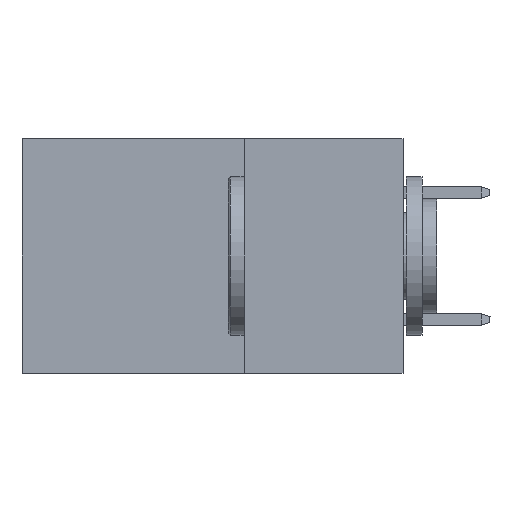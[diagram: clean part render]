
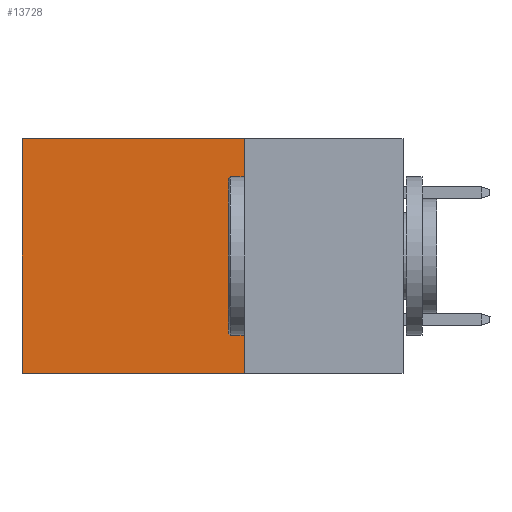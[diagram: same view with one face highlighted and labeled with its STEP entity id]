
A CAD part, left-side view. The second image highlights one B-rep face of the part: STEP entity #13728.
In plain terms, the highlighted planar face has unit normal (-1, 0, 0).
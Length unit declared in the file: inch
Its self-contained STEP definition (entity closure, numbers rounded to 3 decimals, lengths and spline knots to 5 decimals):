
#1766 = ORIENTED_EDGE ( 'NONE', *, *, #11098, .T. ) ;
#2034 = LINE ( 'NONE', #6676, #17856 ) ;
#2366 = ORIENTED_EDGE ( 'NONE', *, *, #22495, .F. ) ;
#5580 = VERTEX_POINT ( 'NONE', #10047 ) ;
#5663 = AXIS2_PLACEMENT_3D ( 'NONE', #6120, #18287, #27669 ) ;
#5741 = DIRECTION ( 'NONE',  ( 0., 1., 0. ) ) ;
#6120 = CARTESIAN_POINT ( 'NONE',  ( 0.2875, 0.25, 0. ) ) ;
#6676 = CARTESIAN_POINT ( 'NONE',  ( 0.2875, 0.6, 0. ) ) ;
#7139 = VECTOR ( 'NONE', #5741, 39.37008 ) ;
#10047 = CARTESIAN_POINT ( 'NONE',  ( 0.2875, 0.25, 0. ) ) ;
#10619 = DIRECTION ( 'NONE',  ( 0., 1., 0. ) ) ;
#10963 = LINE ( 'NONE', #20226, #7139 ) ;
#11098 = EDGE_CURVE ( 'NONE', #20920, #16913, #2034, .T. ) ;
#12945 = VERTEX_POINT ( 'NONE', #28646 ) ;
#13728 = ADVANCED_FACE ( 'NONE', ( #27518 ), #27216, .F. ) ;
#13754 = DIRECTION ( 'NONE',  ( 0., 0., -1. ) ) ;
#16913 = VERTEX_POINT ( 'NONE', #22292 ) ;
#17454 = LINE ( 'NONE', #17616, #18159 ) ;
#17616 = CARTESIAN_POINT ( 'NONE',  ( 0.2875, 0.25, 0. ) ) ;
#17856 = VECTOR ( 'NONE', #13754, 39.37008 ) ;
#18140 = ORIENTED_EDGE ( 'NONE', *, *, #28110, .F. ) ;
#18159 = VECTOR ( 'NONE', #19927, 39.37008 ) ;
#18287 = DIRECTION ( 'NONE',  ( 1., 0., 0. ) ) ;
#19743 = EDGE_CURVE ( 'NONE', #5580, #20920, #29868, .T. ) ;
#19927 = DIRECTION ( 'NONE',  ( 0., 0., -1. ) ) ;
#20226 = CARTESIAN_POINT ( 'NONE',  ( 0.2875, 0.25, -0.37 ) ) ;
#20920 = VERTEX_POINT ( 'NONE', #28228 ) ;
#22054 = EDGE_LOOP ( 'NONE', ( #1766, #2366, #18140, #29371 ) ) ;
#22292 = CARTESIAN_POINT ( 'NONE',  ( 0.2875, 0.6, -0.37 ) ) ;
#22495 = EDGE_CURVE ( 'NONE', #12945, #16913, #10963, .T. ) ;
#25534 = VECTOR ( 'NONE', #10619, 39.37008 ) ;
#27216 = PLANE ( 'NONE',  #5663 ) ;
#27518 = FACE_OUTER_BOUND ( 'NONE', #22054, .T. ) ;
#27546 = CARTESIAN_POINT ( 'NONE',  ( 0.2875, 0.25, 0. ) ) ;
#27669 = DIRECTION ( 'NONE',  ( 0., 0., -1. ) ) ;
#28110 = EDGE_CURVE ( 'NONE', #5580, #12945, #17454, .T. ) ;
#28228 = CARTESIAN_POINT ( 'NONE',  ( 0.2875, 0.6, 0. ) ) ;
#28646 = CARTESIAN_POINT ( 'NONE',  ( 0.2875, 0.25, -0.37 ) ) ;
#29371 = ORIENTED_EDGE ( 'NONE', *, *, #19743, .T. ) ;
#29868 = LINE ( 'NONE', #27546, #25534 ) ;
